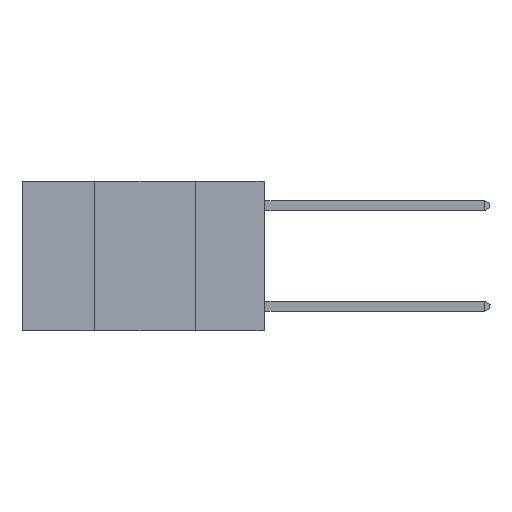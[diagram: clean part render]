
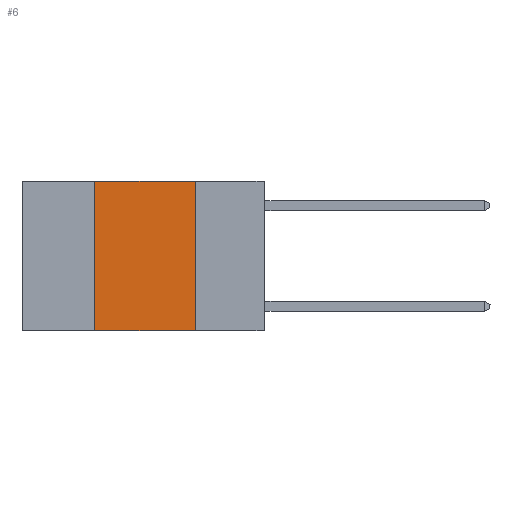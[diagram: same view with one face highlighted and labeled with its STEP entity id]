
A CAD part, left-side view. The second image highlights one B-rep face of the part: STEP entity #6.
In plain terms, the highlighted planar face has unit normal (-1, 0, 0).
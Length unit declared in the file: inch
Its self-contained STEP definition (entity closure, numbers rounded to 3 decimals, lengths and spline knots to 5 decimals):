
#6 = ADVANCED_FACE ( 'NONE', ( #3218 ), #6414, .F. ) ;
#216 = ORIENTED_EDGE ( 'NONE', *, *, #9368, .T. ) ;
#1509 = LINE ( 'NONE', #4124, #7451 ) ;
#2014 = EDGE_CURVE ( 'NONE', #14598, #10252, #1509, .T. ) ;
#3015 = ORIENTED_EDGE ( 'NONE', *, *, #6126, .F. ) ;
#3069 = VECTOR ( 'NONE', #4877, 39.37008 ) ;
#3133 = CARTESIAN_POINT ( 'NONE',  ( 0., 0.6, 0. ) ) ;
#3218 = FACE_OUTER_BOUND ( 'NONE', #14524, .T. ) ;
#3219 = CARTESIAN_POINT ( 'NONE',  ( 0., 0.42, -0.37 ) ) ;
#3350 = DIRECTION ( 'NONE',  ( 0., -1., 0. ) ) ;
#3427 = LINE ( 'NONE', #14247, #3069 ) ;
#3971 = DIRECTION ( 'NONE',  ( 0., 0., -1. ) ) ;
#4124 = CARTESIAN_POINT ( 'NONE',  ( 0., 0.42, 0. ) ) ;
#4307 = DIRECTION ( 'NONE',  ( 0., -1., 0. ) ) ;
#4877 = DIRECTION ( 'NONE',  ( 0., 0., -1. ) ) ;
#5088 = CARTESIAN_POINT ( 'NONE',  ( 0., 0.42, 0. ) ) ;
#5155 = CARTESIAN_POINT ( 'NONE',  ( 0., 0.6, 0. ) ) ;
#5354 = DIRECTION ( 'NONE',  ( 0., 0., 1. ) ) ;
#6126 = EDGE_CURVE ( 'NONE', #11672, #14401, #3427, .T. ) ;
#6414 = PLANE ( 'NONE',  #13691 ) ;
#6534 = EDGE_CURVE ( 'NONE', #10252, #11672, #13230, .T. ) ;
#7451 = VECTOR ( 'NONE', #5354, 39.37008 ) ;
#9306 = ORIENTED_EDGE ( 'NONE', *, *, #6534, .F. ) ;
#9368 = EDGE_CURVE ( 'NONE', #14598, #14401, #11660, .T. ) ;
#10094 = VECTOR ( 'NONE', #4307, 39.37008 ) ;
#10252 = VERTEX_POINT ( 'NONE', #5088 ) ;
#11068 = DIRECTION ( 'NONE',  ( 1., 0., 0. ) ) ;
#11634 = CARTESIAN_POINT ( 'NONE',  ( 0., 0.6, -0.37 ) ) ;
#11660 = LINE ( 'NONE', #11634, #14771 ) ;
#11672 = VERTEX_POINT ( 'NONE', #12871 ) ;
#12456 = ORIENTED_EDGE ( 'NONE', *, *, #2014, .F. ) ;
#12871 = CARTESIAN_POINT ( 'NONE',  ( 0., 0.17, 0. ) ) ;
#13230 = LINE ( 'NONE', #3133, #10094 ) ;
#13459 = CARTESIAN_POINT ( 'NONE',  ( 0., 0.17, -0.37 ) ) ;
#13691 = AXIS2_PLACEMENT_3D ( 'NONE', #5155, #11068, #3971 ) ;
#14247 = CARTESIAN_POINT ( 'NONE',  ( 0., 0.17, 0. ) ) ;
#14401 = VERTEX_POINT ( 'NONE', #13459 ) ;
#14524 = EDGE_LOOP ( 'NONE', ( #3015, #9306, #12456, #216 ) ) ;
#14598 = VERTEX_POINT ( 'NONE', #3219 ) ;
#14771 = VECTOR ( 'NONE', #3350, 39.37008 ) ;
